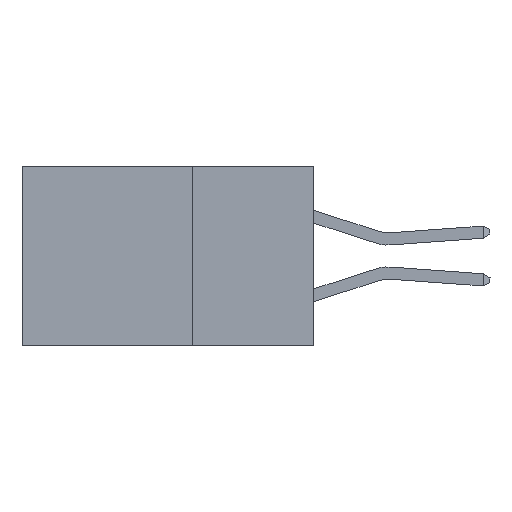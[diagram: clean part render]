
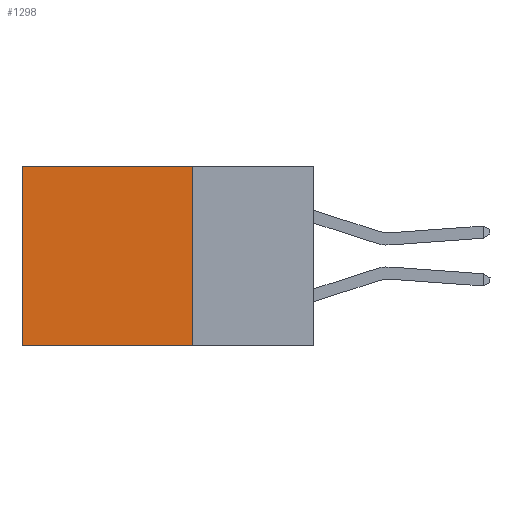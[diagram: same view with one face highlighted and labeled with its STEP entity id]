
A CAD part, left-side view. The second image highlights one B-rep face of the part: STEP entity #1298.
In plain terms, the highlighted planar face has unit normal (-1, 0, 0).
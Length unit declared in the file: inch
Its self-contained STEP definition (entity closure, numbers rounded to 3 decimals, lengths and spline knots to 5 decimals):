
#1011 = VERTEX_POINT ( 'NONE', #18933 ) ;
#1298 = ADVANCED_FACE ( 'NONE', ( #11957 ), #10994, .F. ) ;
#2571 = CARTESIAN_POINT ( 'NONE',  ( 0.2875, 0.6, -0.37 ) ) ;
#2734 = ORIENTED_EDGE ( 'NONE', *, *, #19910, .F. ) ;
#2926 = VECTOR ( 'NONE', #17001, 39.37008 ) ;
#3409 = VERTEX_POINT ( 'NONE', #8078 ) ;
#4810 = VECTOR ( 'NONE', #12040, 39.37008 ) ;
#4841 = VERTEX_POINT ( 'NONE', #6910 ) ;
#5272 = CARTESIAN_POINT ( 'NONE',  ( 0.2875, 0.25, -0.37 ) ) ;
#5914 = CARTESIAN_POINT ( 'NONE',  ( 0.2875, 0.25, 0. ) ) ;
#6762 = LINE ( 'NONE', #22194, #20033 ) ;
#6910 = CARTESIAN_POINT ( 'NONE',  ( 0.2875, 0.25, -0.37 ) ) ;
#7481 = LINE ( 'NONE', #15210, #2926 ) ;
#7875 = EDGE_LOOP ( 'NONE', ( #10895, #2734, #20018, #21334 ) ) ;
#8078 = CARTESIAN_POINT ( 'NONE',  ( 0.2875, 0.6, 0. ) ) ;
#9150 = CARTESIAN_POINT ( 'NONE',  ( 0.2875, 0.6, 0. ) ) ;
#9257 = EDGE_CURVE ( 'NONE', #1011, #3409, #6762, .T. ) ;
#9362 = DIRECTION ( 'NONE',  ( 1., 0., 0. ) ) ;
#10895 = ORIENTED_EDGE ( 'NONE', *, *, #16306, .T. ) ;
#10994 = PLANE ( 'NONE',  #15392 ) ;
#11957 = FACE_OUTER_BOUND ( 'NONE', #7875, .T. ) ;
#12040 = DIRECTION ( 'NONE',  ( 0., 1., 0. ) ) ;
#13282 = VECTOR ( 'NONE', #14233, 39.37008 ) ;
#14233 = DIRECTION ( 'NONE',  ( 0., 0., -1. ) ) ;
#14780 = EDGE_CURVE ( 'NONE', #1011, #4841, #7481, .T. ) ;
#15210 = CARTESIAN_POINT ( 'NONE',  ( 0.2875, 0.25, 0. ) ) ;
#15392 = AXIS2_PLACEMENT_3D ( 'NONE', #5914, #9362, #21494 ) ;
#16036 = LINE ( 'NONE', #9150, #13282 ) ;
#16306 = EDGE_CURVE ( 'NONE', #3409, #16397, #16036, .T. ) ;
#16397 = VERTEX_POINT ( 'NONE', #2571 ) ;
#17001 = DIRECTION ( 'NONE',  ( 0., 0., -1. ) ) ;
#18028 = LINE ( 'NONE', #5272, #4810 ) ;
#18933 = CARTESIAN_POINT ( 'NONE',  ( 0.2875, 0.25, 0. ) ) ;
#19910 = EDGE_CURVE ( 'NONE', #4841, #16397, #18028, .T. ) ;
#20018 = ORIENTED_EDGE ( 'NONE', *, *, #14780, .F. ) ;
#20033 = VECTOR ( 'NONE', #20453, 39.37008 ) ;
#20453 = DIRECTION ( 'NONE',  ( 0., 1., 0. ) ) ;
#21334 = ORIENTED_EDGE ( 'NONE', *, *, #9257, .T. ) ;
#21494 = DIRECTION ( 'NONE',  ( 0., 0., -1. ) ) ;
#22194 = CARTESIAN_POINT ( 'NONE',  ( 0.2875, 0.25, 0. ) ) ;
